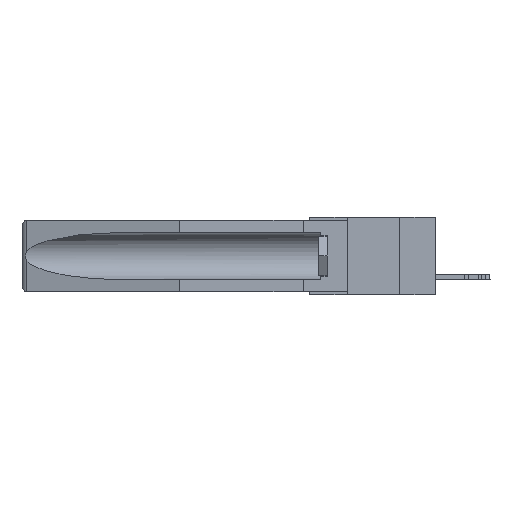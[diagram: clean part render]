
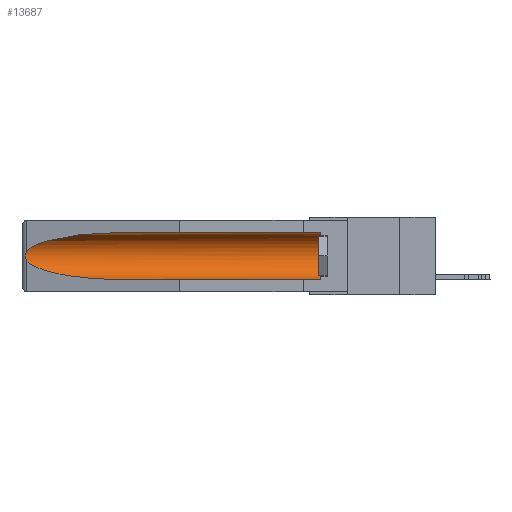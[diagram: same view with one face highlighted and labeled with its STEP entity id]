
A CAD part, left-side view. The second image highlights one B-rep face of the part: STEP entity #13687.
In plain terms, the highlighted cylindrical face has radius 2.857 mm (diameter 5.715 mm), a partial arc.
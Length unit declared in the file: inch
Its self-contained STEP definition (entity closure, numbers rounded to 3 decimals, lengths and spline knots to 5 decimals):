
#305 = CARTESIAN_POINT ( 'NONE',  ( 0.26537, 1.52718, -0.14972 ) ) ;
#327 = EDGE_CURVE ( 'NONE', #3967, #14887, #25980, .T. ) ;
#681 = CARTESIAN_POINT ( 'NONE',  ( 0.21114, 1.30732, -0.284 ) ) ;
#1208 = CARTESIAN_POINT ( 'NONE',  ( 0.155, 1.07973, -0.059 ) ) ;
#2054 =( BOUNDED_CURVE ( )  B_SPLINE_CURVE ( 3, ( #1208, #23574, #13357, #3583 ),
 .UNSPECIFIED., .F., .F. ) 
 B_SPLINE_CURVE_WITH_KNOTS ( ( 4, 4 ),
 ( 4.71239, 6.08839 ),
 .UNSPECIFIED. ) 
 CURVE ( )  GEOMETRIC_REPRESENTATION_ITEM ( )  RATIONAL_B_SPLINE_CURVE ( ( 1., 0.848, 0.848, 1. ) ) 
 REPRESENTATION_ITEM ( '' )  );
#2703 = CARTESIAN_POINT ( 'NONE',  ( 0.26597, 1.52961, -0.15275 ) ) ;
#3583 = CARTESIAN_POINT ( 'NONE',  ( 0.26537, 1.52718, -0.14972 ) ) ;
#3854 = ORIENTED_EDGE ( 'NONE', *, *, #15348, .T. ) ;
#3967 = VERTEX_POINT ( 'NONE', #31818 ) ;
#5524 = CARTESIAN_POINT ( 'NONE',  ( 0.26537, 1.52718, -0.19328 ) ) ;
#6332 = DIRECTION ( 'NONE',  ( 0., 1., 0. ) ) ;
#6825 = DIRECTION ( 'NONE',  ( 0., -1., 0. ) ) ;
#6842 = CARTESIAN_POINT ( 'NONE',  ( 0.155, -0.30754, -0.284 ) ) ;
#7148 = DIRECTION ( 'NONE',  ( 0., 0., 1. ) ) ;
#8061 = ORIENTED_EDGE ( 'NONE', *, *, #26745, .T. ) ;
#9296 = FACE_OUTER_BOUND ( 'NONE', #25358, .T. ) ;
#10163 = CARTESIAN_POINT ( 'NONE',  ( 0.26537, 1.52718, -0.19328 ) ) ;
#11111 = VERTEX_POINT ( 'NONE', #19938 ) ;
#12874 = CARTESIAN_POINT ( 'NONE',  ( 0.2675, 1.53308, -0.17534 ) ) ;
#12984 = CARTESIAN_POINT ( 'NONE',  ( 0.2675, 1.53308, -0.16763 ) ) ;
#13357 = CARTESIAN_POINT ( 'NONE',  ( 0.25451, 1.48313, -0.09465 ) ) ;
#13586 = CARTESIAN_POINT ( 'NONE',  ( 0.155, -0.30754, -0.1715 ) ) ;
#13682 = EDGE_CURVE ( 'NONE', #20357, #24355, #17510, .T. ) ;
#13687 = ADVANCED_FACE ( 'NONE', ( #9296 ), #31783, .F. ) ;
#14377 = ORIENTED_EDGE ( 'NONE', *, *, #327, .T. ) ;
#14608 = CARTESIAN_POINT ( 'NONE',  ( 0.155, 0.126, -0.1715 ) ) ;
#14887 = VERTEX_POINT ( 'NONE', #19080 ) ;
#15279 = CARTESIAN_POINT ( 'NONE',  ( 0.26655, 1.53094, -0.18657 ) ) ;
#15348 = EDGE_CURVE ( 'NONE', #14887, #11111, #23376, .T. ) ;
#15607 = CARTESIAN_POINT ( 'NONE',  ( 0.26654, 1.53092, -0.15636 ) ) ;
#15681 = ORIENTED_EDGE ( 'NONE', *, *, #30260, .T. ) ;
#16087 = B_SPLINE_CURVE_WITH_KNOTS ( 'NONE', 3,
 ( #305, #2703, #15607, #22773, #12984, #12874, #18044, #15279, #18149, #5524 ),
 .UNSPECIFIED., .F., .F.,
 ( 4, 2, 2, 2, 4 ),
 ( 0., 0.00029, 0.00058, 0.00087, 0.00117 ),
 .UNSPECIFIED. ) ;
#17510 =( BOUNDED_CURVE ( )  B_SPLINE_CURVE ( 3, ( #24896, #30082, #681, #31415 ),
 .UNSPECIFIED., .F., .F. ) 
 B_SPLINE_CURVE_WITH_KNOTS ( ( 4, 4 ),
 ( 0.1948, 1.5708 ),
 .UNSPECIFIED. ) 
 CURVE ( )  GEOMETRIC_REPRESENTATION_ITEM ( )  RATIONAL_B_SPLINE_CURVE ( ( 1., 0.848, 0.848, 1. ) ) 
 REPRESENTATION_ITEM ( '' )  );
#18044 = CARTESIAN_POINT ( 'NONE',  ( 0.2673, 1.53269, -0.17917 ) ) ;
#18149 = CARTESIAN_POINT ( 'NONE',  ( 0.26597, 1.5296, -0.19026 ) ) ;
#19080 = CARTESIAN_POINT ( 'NONE',  ( 0.155, 0.126, -0.059 ) ) ;
#19746 = EDGE_CURVE ( 'NONE', #3967, #24355, #30937, .T. ) ;
#19938 = CARTESIAN_POINT ( 'NONE',  ( 0.155, 1.07973, -0.059 ) ) ;
#20357 = VERTEX_POINT ( 'NONE', #10163 ) ;
#21106 = AXIS2_PLACEMENT_3D ( 'NONE', #13586, #6332, #26422 ) ;
#21588 = DIRECTION ( 'NONE',  ( 0., 1., 0. ) ) ;
#22773 = CARTESIAN_POINT ( 'NONE',  ( 0.2673, 1.5327, -0.16383 ) ) ;
#23376 = LINE ( 'NONE', #24171, #24182 ) ;
#23574 = CARTESIAN_POINT ( 'NONE',  ( 0.21114, 1.30732, -0.059 ) ) ;
#24084 = ORIENTED_EDGE ( 'NONE', *, *, #19746, .F. ) ;
#24171 = CARTESIAN_POINT ( 'NONE',  ( 0.155, -0.30754, -0.059 ) ) ;
#24182 = VECTOR ( 'NONE', #24279, 39.37008 ) ;
#24279 = DIRECTION ( 'NONE',  ( 0., 1., 0. ) ) ;
#24355 = VERTEX_POINT ( 'NONE', #27510 ) ;
#24653 = ORIENTED_EDGE ( 'NONE', *, *, #13682, .T. ) ;
#24896 = CARTESIAN_POINT ( 'NONE',  ( 0.26537, 1.52718, -0.19328 ) ) ;
#25358 = EDGE_LOOP ( 'NONE', ( #15681, #8061, #24653, #24084, #14377, #3854 ) ) ;
#25980 = CIRCLE ( 'NONE', #29304, 0.1125 ) ;
#26422 = DIRECTION ( 'NONE',  ( 0., 0., 1. ) ) ;
#26745 = EDGE_CURVE ( 'NONE', #28787, #20357, #16087, .T. ) ;
#27510 = CARTESIAN_POINT ( 'NONE',  ( 0.155, 1.07973, -0.284 ) ) ;
#28787 = VERTEX_POINT ( 'NONE', #31873 ) ;
#29304 = AXIS2_PLACEMENT_3D ( 'NONE', #14608, #6825, #7148 ) ;
#30082 = CARTESIAN_POINT ( 'NONE',  ( 0.25451, 1.48313, -0.24835 ) ) ;
#30260 = EDGE_CURVE ( 'NONE', #11111, #28787, #2054, .T. ) ;
#30937 = LINE ( 'NONE', #6842, #32104 ) ;
#31415 = CARTESIAN_POINT ( 'NONE',  ( 0.155, 1.07973, -0.284 ) ) ;
#31783 = CYLINDRICAL_SURFACE ( 'NONE', #21106, 0.1125 ) ;
#31818 = CARTESIAN_POINT ( 'NONE',  ( 0.155, 0.126, -0.284 ) ) ;
#31873 = CARTESIAN_POINT ( 'NONE',  ( 0.26537, 1.52718, -0.14972 ) ) ;
#32104 = VECTOR ( 'NONE', #21588, 39.37008 ) ;
